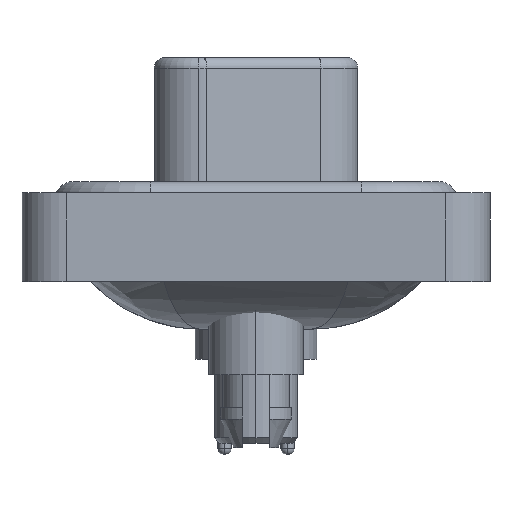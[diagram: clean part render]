
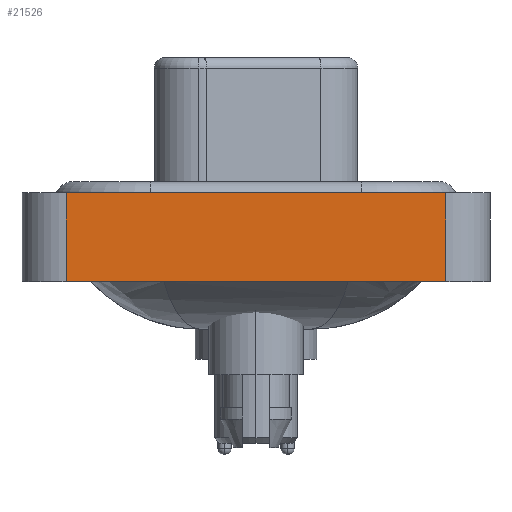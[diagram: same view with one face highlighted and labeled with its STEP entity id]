
A CAD part, left-side view. The second image highlights one B-rep face of the part: STEP entity #21526.
In plain terms, the highlighted planar face has unit normal (-1, 0, 0).
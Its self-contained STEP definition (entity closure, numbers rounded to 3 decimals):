
#649 = LINE ( 'NONE', #11708, #26147 ) ;
#1109 = VERTEX_POINT ( 'NONE', #1458 ) ;
#1458 = CARTESIAN_POINT ( 'NONE',  ( -7.35, 8.55, 0.4 ) ) ;
#1670 = FACE_OUTER_BOUND ( 'NONE', #19777, .T. ) ;
#2116 = DIRECTION ( 'NONE',  ( 0., 0., 1. ) ) ;
#2508 = ORIENTED_EDGE ( 'NONE', *, *, #14368, .F. ) ;
#3187 = CARTESIAN_POINT ( 'NONE',  ( -7.35, 8.55, -3.6 ) ) ;
#3225 = VERTEX_POINT ( 'NONE', #17319 ) ;
#3796 = EDGE_CURVE ( 'NONE', #22221, #26876, #649, .T. ) ;
#3984 = ORIENTED_EDGE ( 'NONE', *, *, #9358, .F. ) ;
#4002 = ORIENTED_EDGE ( 'NONE', *, *, #3796, .T. ) ;
#5037 = DIRECTION ( 'NONE',  ( 0., 0., 1. ) ) ;
#7969 = DIRECTION ( 'NONE',  ( 0., -1., 0. ) ) ;
#8426 = VECTOR ( 'NONE', #5037, 1000. ) ;
#8704 = VECTOR ( 'NONE', #7969, 1000. ) ;
#9358 = EDGE_CURVE ( 'NONE', #1109, #3225, #14217, .T. ) ;
#9587 = DIRECTION ( 'NONE',  ( 0., -1., 0. ) ) ;
#10737 = DIRECTION ( 'NONE',  ( 0., 0., 1. ) ) ;
#11051 = AXIS2_PLACEMENT_3D ( 'NONE', #17026, #25521, #10737 ) ;
#11708 = CARTESIAN_POINT ( 'NONE',  ( -7.35, -8.55, -3.6 ) ) ;
#14217 = LINE ( 'NONE', #20595, #8704 ) ;
#14368 = EDGE_CURVE ( 'NONE', #22221, #1109, #25827, .T. ) ;
#14730 = ORIENTED_EDGE ( 'NONE', *, *, #24286, .T. ) ;
#15840 = LINE ( 'NONE', #24468, #8426 ) ;
#17026 = CARTESIAN_POINT ( 'NONE',  ( -7.35, -8.55, -3.6 ) ) ;
#17319 = CARTESIAN_POINT ( 'NONE',  ( -7.35, -8.55, 0.4 ) ) ;
#18411 = CARTESIAN_POINT ( 'NONE',  ( -7.35, -8.55, -3.6 ) ) ;
#18987 = PLANE ( 'NONE',  #11051 ) ;
#19777 = EDGE_LOOP ( 'NONE', ( #14730, #3984, #2508, #4002 ) ) ;
#20595 = CARTESIAN_POINT ( 'NONE',  ( -7.35, -8.55, 0.4 ) ) ;
#21526 = ADVANCED_FACE ( 'NONE', ( #1670 ), #18987, .T. ) ;
#22221 = VERTEX_POINT ( 'NONE', #3187 ) ;
#24286 = EDGE_CURVE ( 'NONE', #26876, #3225, #15840, .T. ) ;
#24468 = CARTESIAN_POINT ( 'NONE',  ( -7.35, -8.55, -3.6 ) ) ;
#25520 = VECTOR ( 'NONE', #2116, 1000. ) ;
#25521 = DIRECTION ( 'NONE',  ( -1., 0., 0. ) ) ;
#25827 = LINE ( 'NONE', #26103, #25520 ) ;
#26103 = CARTESIAN_POINT ( 'NONE',  ( -7.35, 8.55, -3.6 ) ) ;
#26147 = VECTOR ( 'NONE', #9587, 1000. ) ;
#26876 = VERTEX_POINT ( 'NONE', #18411 ) ;
